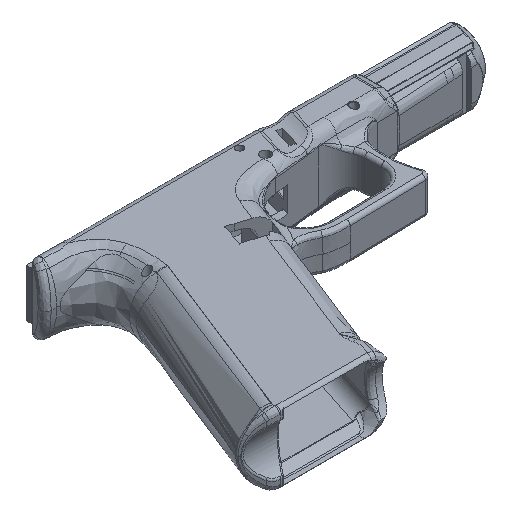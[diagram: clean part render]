
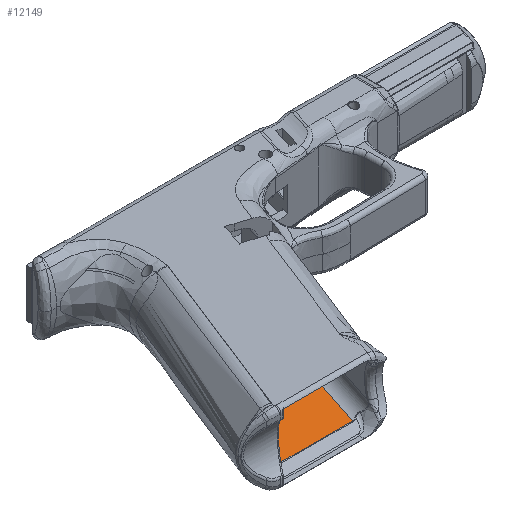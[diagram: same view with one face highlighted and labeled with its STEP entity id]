
A CAD part, isometric view. The second image highlights one B-rep face of the part: STEP entity #12149.
In plain terms, the highlighted planar face has unit normal (0, 0, 1).
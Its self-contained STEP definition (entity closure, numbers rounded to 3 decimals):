
#1838=FACE_OUTER_BOUND('',#2535,.T.);
#2535=EDGE_LOOP('',(#8560,#8561,#8562,#8563,#8564,#8565,#8566,#8567,#8568,
#8569,#8570,#8571,#8572));
#3143=LINE('',#17745,#3872);
#3189=LINE('',#22071,#3918);
#3206=LINE('',#23869,#3935);
#3212=LINE('',#23881,#3941);
#3213=LINE('',#23883,#3942);
#3214=LINE('',#23885,#3943);
#3215=LINE('',#23887,#3944);
#3216=LINE('',#23889,#3945);
#3217=LINE('',#23891,#3946);
#3218=LINE('',#23893,#3947);
#3219=LINE('',#23895,#3948);
#3220=LINE('',#23897,#3949);
#3221=LINE('',#23898,#3950);
#3872=VECTOR('',#13863,10.);
#3918=VECTOR('',#14107,10.);
#3935=VECTOR('',#14174,10.);
#3941=VECTOR('',#14182,10.);
#3942=VECTOR('',#14183,1000.);
#3943=VECTOR('',#14184,10.);
#3944=VECTOR('',#14185,10.);
#3945=VECTOR('',#14186,10.);
#3946=VECTOR('',#14187,10.);
#3947=VECTOR('',#14188,10.);
#3948=VECTOR('',#14189,10.);
#3949=VECTOR('',#14190,10.);
#3950=VECTOR('',#14191,10.);
#4816=VERTEX_POINT('',#17734);
#4820=VERTEX_POINT('',#17744);
#4949=VERTEX_POINT('',#22068);
#4988=VERTEX_POINT('',#23868);
#4993=VERTEX_POINT('',#23880);
#4994=VERTEX_POINT('',#23882);
#4995=VERTEX_POINT('',#23884);
#4996=VERTEX_POINT('',#23886);
#4997=VERTEX_POINT('',#23888);
#4998=VERTEX_POINT('',#23890);
#4999=VERTEX_POINT('',#23892);
#5000=VERTEX_POINT('',#23894);
#5001=VERTEX_POINT('',#23896);
#6076=EDGE_CURVE('',#4816,#4820,#3143,.T.);
#6279=EDGE_CURVE('',#4820,#4949,#3189,.T.);
#6338=EDGE_CURVE('',#4949,#4988,#3206,.T.);
#6344=EDGE_CURVE('',#4993,#4816,#3212,.T.);
#6345=EDGE_CURVE('',#4993,#4994,#3213,.T.);
#6346=EDGE_CURVE('',#4994,#4995,#3214,.T.);
#6347=EDGE_CURVE('',#4996,#4995,#3215,.F.);
#6348=EDGE_CURVE('',#4997,#4996,#3216,.F.);
#6349=EDGE_CURVE('',#4998,#4997,#3217,.F.);
#6350=EDGE_CURVE('',#4999,#4998,#3218,.F.);
#6351=EDGE_CURVE('',#5000,#4999,#3219,.F.);
#6352=EDGE_CURVE('',#5001,#5000,#3220,.F.);
#6353=EDGE_CURVE('',#4988,#5001,#3221,.T.);
#8560=ORIENTED_EDGE('',*,*,#6279,.F.);
#8561=ORIENTED_EDGE('',*,*,#6076,.F.);
#8562=ORIENTED_EDGE('',*,*,#6344,.F.);
#8563=ORIENTED_EDGE('',*,*,#6345,.T.);
#8564=ORIENTED_EDGE('',*,*,#6346,.T.);
#8565=ORIENTED_EDGE('',*,*,#6347,.F.);
#8566=ORIENTED_EDGE('',*,*,#6348,.F.);
#8567=ORIENTED_EDGE('',*,*,#6349,.F.);
#8568=ORIENTED_EDGE('',*,*,#6350,.F.);
#8569=ORIENTED_EDGE('',*,*,#6351,.F.);
#8570=ORIENTED_EDGE('',*,*,#6352,.F.);
#8571=ORIENTED_EDGE('',*,*,#6353,.F.);
#8572=ORIENTED_EDGE('',*,*,#6338,.F.);
#11855=PLANE('',#12909);
#12149=ADVANCED_FACE('',(#1838),#11855,.T.);
#12909=AXIS2_PLACEMENT_3D('',#23879,#14180,#14181);
#13863=DIRECTION('',(-1.,0.,0.));
#14107=DIRECTION('',(0.309,0.951,0.));
#14174=DIRECTION('',(0.309,0.951,0.));
#14180=DIRECTION('center_axis',(0.,0.,1.));
#14181=DIRECTION('ref_axis',(1.,0.,0.));
#14182=DIRECTION('',(-0.309,-0.951,0.));
#14183=DIRECTION('',(1.,0.,0.));
#14184=DIRECTION('',(0.301,0.954,0.));
#14185=DIRECTION('',(-1.,0.,0.));
#14186=DIRECTION('',(0.,-1.,0.));
#14187=DIRECTION('',(-1.,0.,0.));
#14188=DIRECTION('',(0.,1.,0.));
#14189=DIRECTION('',(-1.,0.,0.));
#14190=DIRECTION('',(-0.309,-0.951,0.));
#14191=DIRECTION('',(0.951,-0.309,0.));
#17734=CARTESIAN_POINT('',(32.909,-97.822,-11.75));
#17744=CARTESIAN_POINT('',(2.294,-97.822,-11.75));
#17745=CARTESIAN_POINT('',(6.8,-97.822,-11.75));
#22068=CARTESIAN_POINT('',(18.552,-47.783,-11.75));
#22071=CARTESIAN_POINT('',(2.312,-97.765,-11.75));
#23868=CARTESIAN_POINT('',(32.169,-5.875,-11.75));
#23869=CARTESIAN_POINT('',(5.462,-88.072,-11.75));
#23879=CARTESIAN_POINT('Origin',(-2.2,-1.,-11.75));
#23880=CARTESIAN_POINT('',(59.494,-16.,-11.75));
#23881=CARTESIAN_POINT('',(43.969,-63.781,-11.75));
#23882=CARTESIAN_POINT('',(65.192,-16.,-11.75));
#23883=CARTESIAN_POINT('',(0.,-16.,-11.75));
#23884=CARTESIAN_POINT('',(69.764,-1.5,-11.75));
#23885=CARTESIAN_POINT('',(66.549,-11.698,-11.75));
#23886=CARTESIAN_POINT('',(62.1,-1.5,-11.75));
#23887=CARTESIAN_POINT('',(61.488,-1.5,-11.75));
#23888=CARTESIAN_POINT('',(62.1,-3.,-11.75));
#23889=CARTESIAN_POINT('',(62.1,-53.999,-11.75));
#23890=CARTESIAN_POINT('',(52.35,-3.,-11.75));
#23891=CARTESIAN_POINT('',(46.014,-3.,-11.75));
#23892=CARTESIAN_POINT('',(52.35,-1.5,-11.75));
#23893=CARTESIAN_POINT('',(52.35,-54.999,-11.75));
#23894=CARTESIAN_POINT('',(47.586,-1.5,-11.75));
#23895=CARTESIAN_POINT('',(61.488,-1.5,-11.75));
#23896=CARTESIAN_POINT('',(44.828,-9.989,-11.75));
#23897=CARTESIAN_POINT('',(29.862,-56.051,-11.75));
#23898=CARTESIAN_POINT('',(32.712,-6.052,-11.75));
